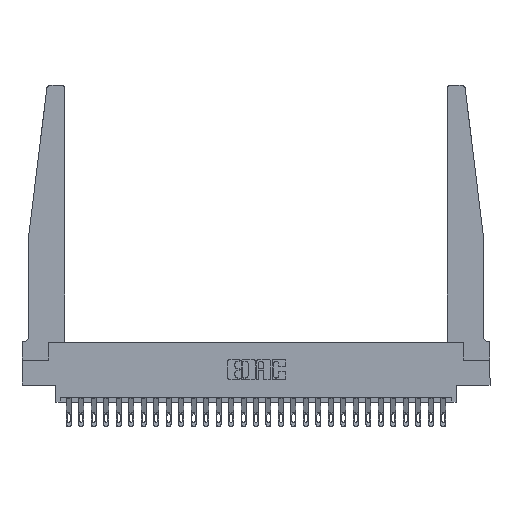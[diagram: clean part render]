
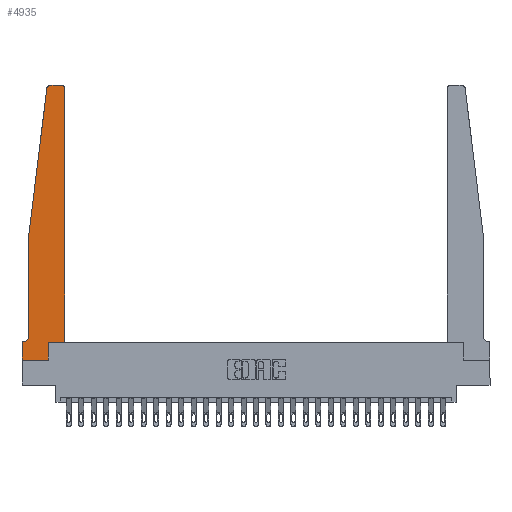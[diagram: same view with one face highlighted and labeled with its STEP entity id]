
A CAD part, top view. The second image highlights one B-rep face of the part: STEP entity #4935.
In plain terms, the highlighted planar face has unit normal (0, 0, 1).
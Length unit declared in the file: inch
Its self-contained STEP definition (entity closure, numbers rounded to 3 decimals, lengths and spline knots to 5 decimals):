
#38 = CARTESIAN_POINT ( 'NONE',  ( 0.425, 0.18, 0.37 ) ) ;
#86 = LINE ( 'NONE', #15164, #26473 ) ;
#347 = EDGE_CURVE ( 'NONE', #9215, #24983, #6485, .T. ) ;
#442 = EDGE_CURVE ( 'NONE', #24983, #21980, #4511, .T. ) ;
#698 = ORIENTED_EDGE ( 'NONE', *, *, #771, .T. ) ;
#771 = EDGE_CURVE ( 'NONE', #12593, #21105, #13314, .T. ) ;
#1581 = LINE ( 'NONE', #14746, #22467 ) ;
#1898 = ORIENTED_EDGE ( 'NONE', *, *, #11627, .T. ) ;
#1912 = VERTEX_POINT ( 'NONE', #24548 ) ;
#2271 = EDGE_LOOP ( 'NONE', ( #19395, #698, #10365, #22199, #9939, #20973, #3417, #2406, #17176, #13989, #1898, #26263 ) ) ;
#2333 = VERTEX_POINT ( 'NONE', #9197 ) ;
#2406 = ORIENTED_EDGE ( 'NONE', *, *, #11524, .T. ) ;
#2511 = EDGE_CURVE ( 'NONE', #2333, #17464, #10140, .T. ) ;
#3051 = CARTESIAN_POINT ( 'NONE',  ( 0.065, 0.2375, 0.37 ) ) ;
#3288 = VERTEX_POINT ( 'NONE', #38 ) ;
#3417 = ORIENTED_EDGE ( 'NONE', *, *, #442, .T. ) ;
#3575 = CARTESIAN_POINT ( 'NONE',  ( 0.27653, 2.72, 0.37 ) ) ;
#3834 = VECTOR ( 'NONE', #13045, 39.37008 ) ;
#4272 = CARTESIAN_POINT ( 'NONE',  ( 0.395, 2.72, 0.37 ) ) ;
#4356 = AXIS2_PLACEMENT_3D ( 'NONE', #7137, #21748, #9237 ) ;
#4386 = DIRECTION ( 'NONE',  ( 1., 0., 0. ) ) ;
#4511 = LINE ( 'NONE', #22955, #14926 ) ;
#4935 = ADVANCED_FACE ( 'NONE', ( #26352 ), #15407, .T. ) ;
#5196 = CIRCLE ( 'NONE', #21854, 0.05 ) ;
#5682 = DIRECTION ( 'NONE',  ( 0., 0., -1. ) ) ;
#6373 = DIRECTION ( 'NONE',  ( 1., 0., 0. ) ) ;
#6485 = LINE ( 'NONE', #26840, #22489 ) ;
#7137 = CARTESIAN_POINT ( 'NONE',  ( 0., 0.1875, 0.37 ) ) ;
#7918 = CARTESIAN_POINT ( 'NONE',  ( 0.27653, 2.75, 0.37 ) ) ;
#7940 = CARTESIAN_POINT ( 'NONE',  ( 0.25, 2.75, 0.37 ) ) ;
#8990 = DIRECTION ( 'NONE',  ( -0.122, -0.992, 0. ) ) ;
#9197 = CARTESIAN_POINT ( 'NONE',  ( 0.2605, 0., 0.37 ) ) ;
#9215 = VERTEX_POINT ( 'NONE', #25176 ) ;
#9237 = DIRECTION ( 'NONE',  ( 1., 0., 0. ) ) ;
#9270 = VECTOR ( 'NONE', #19122, 39.37008 ) ;
#9332 = CARTESIAN_POINT ( 'NONE',  ( 0.2605, 0.18, 0.37 ) ) ;
#9657 = AXIS2_PLACEMENT_3D ( 'NONE', #4272, #18854, #6373 ) ;
#9694 = DIRECTION ( 'NONE',  ( 1., 0., 0. ) ) ;
#9768 = EDGE_CURVE ( 'NONE', #1912, #26943, #24825, .T. ) ;
#9939 = ORIENTED_EDGE ( 'NONE', *, *, #17609, .T. ) ;
#10140 = LINE ( 'NONE', #18395, #21277 ) ;
#10365 = ORIENTED_EDGE ( 'NONE', *, *, #15419, .T. ) ;
#10936 = CARTESIAN_POINT ( 'NONE',  ( 0.425, 0.18, 0.37 ) ) ;
#11319 = CARTESIAN_POINT ( 'NONE',  ( 0., 0., 0.37 ) ) ;
#11524 = EDGE_CURVE ( 'NONE', #21980, #2333, #1581, .T. ) ;
#11627 = EDGE_CURVE ( 'NONE', #3288, #1912, #21139, .T. ) ;
#11722 = CARTESIAN_POINT ( 'NONE',  ( 0., 0.1875, 0.37 ) ) ;
#12593 = VERTEX_POINT ( 'NONE', #7918 ) ;
#13045 = DIRECTION ( 'NONE',  ( 0., 1., 0. ) ) ;
#13095 = DIRECTION ( 'NONE',  ( 1., 0., 0. ) ) ;
#13314 = CIRCLE ( 'NONE', #19129, 0.03 ) ;
#13804 = DIRECTION ( 'NONE',  ( 0., -1., 0. ) ) ;
#13807 = CARTESIAN_POINT ( 'NONE',  ( 0.425, 0.18, 0.37 ) ) ;
#13989 = ORIENTED_EDGE ( 'NONE', *, *, #19290, .T. ) ;
#14523 = VECTOR ( 'NONE', #9694, 39.37008 ) ;
#14746 = CARTESIAN_POINT ( 'NONE',  ( 0., 0., 0.37 ) ) ;
#14926 = VECTOR ( 'NONE', #13804, 39.37008 ) ;
#15063 = EDGE_CURVE ( 'NONE', #26943, #12593, #19015, .T. ) ;
#15164 = CARTESIAN_POINT ( 'NONE',  ( 0.065, 1.25, 0.37 ) ) ;
#15407 = PLANE ( 'NONE',  #4356 ) ;
#15419 = EDGE_CURVE ( 'NONE', #21105, #23361, #86, .T. ) ;
#15974 = CARTESIAN_POINT ( 'NONE',  ( 0.065, 1.25, 0.37 ) ) ;
#17014 = CARTESIAN_POINT ( 'NONE',  ( 0.065, 1.25, 0.37 ) ) ;
#17176 = ORIENTED_EDGE ( 'NONE', *, *, #2511, .T. ) ;
#17450 = VERTEX_POINT ( 'NONE', #3051 ) ;
#17464 = VERTEX_POINT ( 'NONE', #9332 ) ;
#17609 = EDGE_CURVE ( 'NONE', #17450, #9215, #5196, .T. ) ;
#18162 = CARTESIAN_POINT ( 'NONE',  ( 0.015, 0.2375, 0.37 ) ) ;
#18312 = DIRECTION ( 'NONE',  ( -1., 0., 0. ) ) ;
#18372 = VECTOR ( 'NONE', #18312, 39.37008 ) ;
#18395 = CARTESIAN_POINT ( 'NONE',  ( 0.2605, 0.18, 0.37 ) ) ;
#18854 = DIRECTION ( 'NONE',  ( 0., 0., 1. ) ) ;
#19015 = LINE ( 'NONE', #7940, #18372 ) ;
#19122 = DIRECTION ( 'NONE',  ( 0., -1., 0. ) ) ;
#19129 = AXIS2_PLACEMENT_3D ( 'NONE', #3575, #20379, #13095 ) ;
#19290 = EDGE_CURVE ( 'NONE', #17464, #3288, #26277, .T. ) ;
#19395 = ORIENTED_EDGE ( 'NONE', *, *, #15063, .T. ) ;
#20267 = DIRECTION ( 'NONE',  ( -1., 0., 0. ) ) ;
#20363 = LINE ( 'NONE', #17014, #9270 ) ;
#20379 = DIRECTION ( 'NONE',  ( 0., 0., 1. ) ) ;
#20380 = CARTESIAN_POINT ( 'NONE',  ( 0.24675, 2.72367, 0.37 ) ) ;
#20973 = ORIENTED_EDGE ( 'NONE', *, *, #347, .T. ) ;
#21105 = VERTEX_POINT ( 'NONE', #20380 ) ;
#21139 = LINE ( 'NONE', #10936, #3834 ) ;
#21277 = VECTOR ( 'NONE', #24614, 39.37008 ) ;
#21748 = DIRECTION ( 'NONE',  ( 0., 0., 1. ) ) ;
#21854 = AXIS2_PLACEMENT_3D ( 'NONE', #18162, #5682, #20267 ) ;
#21980 = VERTEX_POINT ( 'NONE', #11319 ) ;
#22199 = ORIENTED_EDGE ( 'NONE', *, *, #22456, .T. ) ;
#22456 = EDGE_CURVE ( 'NONE', #23361, #17450, #20363, .T. ) ;
#22467 = VECTOR ( 'NONE', #4386, 39.37008 ) ;
#22489 = VECTOR ( 'NONE', #24146, 39.37008 ) ;
#22955 = CARTESIAN_POINT ( 'NONE',  ( 0., 0., 0.37 ) ) ;
#23361 = VERTEX_POINT ( 'NONE', #15974 ) ;
#24146 = DIRECTION ( 'NONE',  ( -1., 0., 0. ) ) ;
#24548 = CARTESIAN_POINT ( 'NONE',  ( 0.425, 2.72, 0.37 ) ) ;
#24614 = DIRECTION ( 'NONE',  ( 0., 1., 0. ) ) ;
#24825 = CIRCLE ( 'NONE', #9657, 0.03 ) ;
#24983 = VERTEX_POINT ( 'NONE', #11722 ) ;
#25176 = CARTESIAN_POINT ( 'NONE',  ( 0.015, 0.1875, 0.37 ) ) ;
#25186 = CARTESIAN_POINT ( 'NONE',  ( 0.395, 2.75, 0.37 ) ) ;
#26263 = ORIENTED_EDGE ( 'NONE', *, *, #9768, .T. ) ;
#26277 = LINE ( 'NONE', #13807, #14523 ) ;
#26352 = FACE_OUTER_BOUND ( 'NONE', #2271, .T. ) ;
#26473 = VECTOR ( 'NONE', #8990, 39.37008 ) ;
#26840 = CARTESIAN_POINT ( 'NONE',  ( 0.065, 0.1875, 0.37 ) ) ;
#26943 = VERTEX_POINT ( 'NONE', #25186 ) ;
